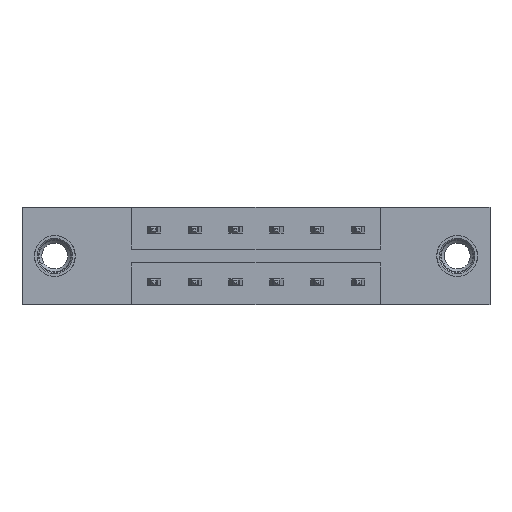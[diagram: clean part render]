
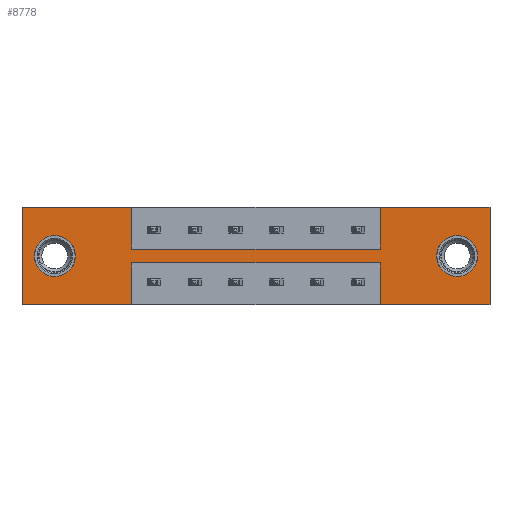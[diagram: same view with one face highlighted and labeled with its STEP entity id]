
A CAD part, front view. The second image highlights one B-rep face of the part: STEP entity #8778.
In plain terms, the highlighted planar face has unit normal (0, -1, 0).
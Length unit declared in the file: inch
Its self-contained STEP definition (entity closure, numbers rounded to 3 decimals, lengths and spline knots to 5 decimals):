
#43 = LINE ( 'NONE', #3060, #4409 ) ;
#208 = VECTOR ( 'NONE', #5693, 39.37008 ) ;
#381 = EDGE_CURVE ( 'NONE', #5767, #5441, #43, .T. ) ;
#435 = FACE_OUTER_BOUND ( 'NONE', #5698, .T. ) ;
#554 = LINE ( 'NONE', #6455, #8464 ) ;
#583 = AXIS2_PLACEMENT_3D ( 'NONE', #6669, #5352, #9686 ) ;
#607 = DIRECTION ( 'NONE',  ( 0., 1., 0. ) ) ;
#630 = CARTESIAN_POINT ( 'NONE',  ( 0., 0., 0. ) ) ;
#822 = ORIENTED_EDGE ( 'NONE', *, *, #4869, .T. ) ;
#967 = VECTOR ( 'NONE', #7931, 39.37008 ) ;
#1008 = AXIS2_PLACEMENT_3D ( 'NONE', #5091, #5903, #8939 ) ;
#1076 = CARTESIAN_POINT ( 'NONE',  ( 0., 0., -0.37 ) ) ;
#1120 = ORIENTED_EDGE ( 'NONE', *, *, #381, .F. ) ;
#1141 = DIRECTION ( 'NONE',  ( 1., 0., 0. ) ) ;
#1148 = LINE ( 'NONE', #6303, #4455 ) ;
#1151 = CARTESIAN_POINT ( 'NONE',  ( 1.3665, 0., -0.1585 ) ) ;
#1163 = CARTESIAN_POINT ( 'NONE',  ( 0.4175, 0., -0.1585 ) ) ;
#1263 = LINE ( 'NONE', #1163, #8132 ) ;
#1305 = VECTOR ( 'NONE', #8753, 39.37008 ) ;
#1425 = LINE ( 'NONE', #3141, #7980 ) ;
#1603 = VECTOR ( 'NONE', #7417, 39.37008 ) ;
#1613 = VERTEX_POINT ( 'NONE', #2608 ) ;
#1787 = VERTEX_POINT ( 'NONE', #630 ) ;
#1839 = CARTESIAN_POINT ( 'NONE',  ( 1.784, 0., -0.37 ) ) ;
#1968 = PLANE ( 'NONE',  #4619 ) ;
#2608 = CARTESIAN_POINT ( 'NONE',  ( 1.3665, 0., -0.1585 ) ) ;
#2634 = VECTOR ( 'NONE', #9454, 39.37008 ) ;
#2713 = CARTESIAN_POINT ( 'NONE',  ( 0., 0., -0.37 ) ) ;
#2823 = VERTEX_POINT ( 'NONE', #6062 ) ;
#2960 = EDGE_CURVE ( 'NONE', #6636, #5767, #1148, .T. ) ;
#3026 = CARTESIAN_POINT ( 'NONE',  ( 0.4175, 0., 0. ) ) ;
#3060 = CARTESIAN_POINT ( 'NONE',  ( 0.4175, 0., -0.2115 ) ) ;
#3124 = VERTEX_POINT ( 'NONE', #8231 ) ;
#3141 = CARTESIAN_POINT ( 'NONE',  ( 1.784, 0., 0. ) ) ;
#3235 = CARTESIAN_POINT ( 'NONE',  ( 0.4175, 0., -0.2115 ) ) ;
#3307 = DIRECTION ( 'NONE',  ( -1., 0., 0. ) ) ;
#3402 = CARTESIAN_POINT ( 'NONE',  ( 0., 0., 0. ) ) ;
#3451 = EDGE_LOOP ( 'NONE', ( #822, #3766 ) ) ;
#3481 = DIRECTION ( 'NONE',  ( 0., 0., 1. ) ) ;
#3496 = EDGE_CURVE ( 'NONE', #5668, #1787, #5848, .T. ) ;
#3550 = LINE ( 'NONE', #7162, #2634 ) ;
#3578 = DIRECTION ( 'NONE',  ( 0., 0., -1. ) ) ;
#3601 = ORIENTED_EDGE ( 'NONE', *, *, #7201, .F. ) ;
#3766 = ORIENTED_EDGE ( 'NONE', *, *, #4940, .T. ) ;
#3806 = EDGE_CURVE ( 'NONE', #1787, #6797, #4154, .T. ) ;
#3820 = CARTESIAN_POINT ( 'NONE',  ( 1.659, 0., -0.107 ) ) ;
#3928 = EDGE_CURVE ( 'NONE', #4126, #4663, #9031, .T. ) ;
#4056 = DIRECTION ( 'NONE',  ( 0., 0., -1. ) ) ;
#4126 = VERTEX_POINT ( 'NONE', #7000 ) ;
#4154 = LINE ( 'NONE', #3402, #1305 ) ;
#4203 = ORIENTED_EDGE ( 'NONE', *, *, #7881, .F. ) ;
#4241 = ORIENTED_EDGE ( 'NONE', *, *, #3806, .F. ) ;
#4319 = VERTEX_POINT ( 'NONE', #1839 ) ;
#4409 = VECTOR ( 'NONE', #3307, 39.37008 ) ;
#4455 = VECTOR ( 'NONE', #3481, 39.37008 ) ;
#4562 = ORIENTED_EDGE ( 'NONE', *, *, #3496, .F. ) ;
#4619 = AXIS2_PLACEMENT_3D ( 'NONE', #2713, #9515, #7173 ) ;
#4663 = VERTEX_POINT ( 'NONE', #3820 ) ;
#4869 = EDGE_CURVE ( 'NONE', #3124, #9203, #6033, .T. ) ;
#4935 = CARTESIAN_POINT ( 'NONE',  ( 0., 0., -0.37 ) ) ;
#4940 = EDGE_CURVE ( 'NONE', #9203, #3124, #6974, .T. ) ;
#4962 = CARTESIAN_POINT ( 'NONE',  ( 1.3665, 0., -0.37 ) ) ;
#4986 = ORIENTED_EDGE ( 'NONE', *, *, #8275, .F. ) ;
#5003 = CIRCLE ( 'NONE', #583, 0.078 ) ;
#5006 = VERTEX_POINT ( 'NONE', #6187 ) ;
#5091 = CARTESIAN_POINT ( 'NONE',  ( 0.125, 0., -0.185 ) ) ;
#5157 = ORIENTED_EDGE ( 'NONE', *, *, #7501, .T. ) ;
#5194 = EDGE_CURVE ( 'NONE', #6797, #2823, #6465, .T. ) ;
#5225 = ORIENTED_EDGE ( 'NONE', *, *, #8699, .F. ) ;
#5267 = CARTESIAN_POINT ( 'NONE',  ( 0., 0., 0. ) ) ;
#5352 = DIRECTION ( 'NONE',  ( 0., 1., 0. ) ) ;
#5441 = VERTEX_POINT ( 'NONE', #3235 ) ;
#5470 = CARTESIAN_POINT ( 'NONE',  ( 0.4175, 0., -0.1585 ) ) ;
#5647 = DIRECTION ( 'NONE',  ( 1., 0., 0. ) ) ;
#5668 = VERTEX_POINT ( 'NONE', #4935 ) ;
#5680 = CARTESIAN_POINT ( 'NONE',  ( 0.4175, 0., -0.37 ) ) ;
#5693 = DIRECTION ( 'NONE',  ( 0., 0., -1. ) ) ;
#5698 = EDGE_LOOP ( 'NONE', ( #6883, #6481, #3601, #4986, #7463, #6211, #7692, #4241, #4562, #5225, #4203, #1120 ) ) ;
#5767 = VERTEX_POINT ( 'NONE', #9511 ) ;
#5848 = LINE ( 'NONE', #5267, #1603 ) ;
#5858 = DIRECTION ( 'NONE',  ( 0., 0., 1. ) ) ;
#5903 = DIRECTION ( 'NONE',  ( 0., 1., 0. ) ) ;
#5970 = DIRECTION ( 'NONE',  ( 0., 0., -1. ) ) ;
#6025 = CARTESIAN_POINT ( 'NONE',  ( 1.659, 0., -0.185 ) ) ;
#6033 = CIRCLE ( 'NONE', #9514, 0.078 ) ;
#6062 = CARTESIAN_POINT ( 'NONE',  ( 0.4175, 0., -0.1585 ) ) ;
#6187 = CARTESIAN_POINT ( 'NONE',  ( 1.3665, 0., 0. ) ) ;
#6211 = ORIENTED_EDGE ( 'NONE', *, *, #7389, .F. ) ;
#6303 = CARTESIAN_POINT ( 'NONE',  ( 1.3665, 0., -0.2115 ) ) ;
#6318 = AXIS2_PLACEMENT_3D ( 'NONE', #6025, #607, #5970 ) ;
#6433 = LINE ( 'NONE', #1076, #967 ) ;
#6455 = CARTESIAN_POINT ( 'NONE',  ( 0.4175, 0., -0.2115 ) ) ;
#6465 = LINE ( 'NONE', #5470, #208 ) ;
#6481 = ORIENTED_EDGE ( 'NONE', *, *, #7337, .F. ) ;
#6536 = CARTESIAN_POINT ( 'NONE',  ( 0.125, 0., -0.185 ) ) ;
#6601 = EDGE_CURVE ( 'NONE', #1613, #5006, #7903, .T. ) ;
#6636 = VERTEX_POINT ( 'NONE', #4962 ) ;
#6669 = CARTESIAN_POINT ( 'NONE',  ( 1.659, 0., -0.185 ) ) ;
#6691 = DIRECTION ( 'NONE',  ( 0., 1., 0. ) ) ;
#6797 = VERTEX_POINT ( 'NONE', #3026 ) ;
#6883 = ORIENTED_EDGE ( 'NONE', *, *, #2960, .F. ) ;
#6974 = CIRCLE ( 'NONE', #1008, 0.078 ) ;
#7000 = CARTESIAN_POINT ( 'NONE',  ( 1.659, 0., -0.263 ) ) ;
#7070 = FACE_BOUND ( 'NONE', #3451, .T. ) ;
#7083 = LINE ( 'NONE', #8783, #9254 ) ;
#7162 = CARTESIAN_POINT ( 'NONE',  ( 0., 0., -0.37 ) ) ;
#7173 = DIRECTION ( 'NONE',  ( 0., 0., -1. ) ) ;
#7174 = EDGE_LOOP ( 'NONE', ( #5157, #7415 ) ) ;
#7201 = EDGE_CURVE ( 'NONE', #8276, #4319, #1425, .T. ) ;
#7337 = EDGE_CURVE ( 'NONE', #4319, #6636, #3550, .T. ) ;
#7389 = EDGE_CURVE ( 'NONE', #2823, #1613, #1263, .T. ) ;
#7415 = ORIENTED_EDGE ( 'NONE', *, *, #3928, .T. ) ;
#7417 = DIRECTION ( 'NONE',  ( 0., 0., 1. ) ) ;
#7463 = ORIENTED_EDGE ( 'NONE', *, *, #6601, .F. ) ;
#7501 = EDGE_CURVE ( 'NONE', #4663, #4126, #5003, .T. ) ;
#7692 = ORIENTED_EDGE ( 'NONE', *, *, #5194, .F. ) ;
#7817 = VERTEX_POINT ( 'NONE', #5680 ) ;
#7881 = EDGE_CURVE ( 'NONE', #5441, #7817, #554, .T. ) ;
#7903 = LINE ( 'NONE', #1151, #8437 ) ;
#7931 = DIRECTION ( 'NONE',  ( -1., 0., 0. ) ) ;
#7980 = VECTOR ( 'NONE', #4056, 39.37008 ) ;
#8132 = VECTOR ( 'NONE', #5647, 39.37008 ) ;
#8231 = CARTESIAN_POINT ( 'NONE',  ( 0.125, 0., -0.107 ) ) ;
#8275 = EDGE_CURVE ( 'NONE', #5006, #8276, #7083, .T. ) ;
#8276 = VERTEX_POINT ( 'NONE', #9476 ) ;
#8437 = VECTOR ( 'NONE', #8748, 39.37008 ) ;
#8464 = VECTOR ( 'NONE', #3578, 39.37008 ) ;
#8699 = EDGE_CURVE ( 'NONE', #7817, #5668, #6433, .T. ) ;
#8748 = DIRECTION ( 'NONE',  ( 0., 0., 1. ) ) ;
#8753 = DIRECTION ( 'NONE',  ( 1., 0., 0. ) ) ;
#8778 = ADVANCED_FACE ( 'NONE', ( #9328, #7070, #435 ), #1968, .T. ) ;
#8783 = CARTESIAN_POINT ( 'NONE',  ( 0., 0., 0. ) ) ;
#8939 = DIRECTION ( 'NONE',  ( 0., 0., 1. ) ) ;
#9031 = CIRCLE ( 'NONE', #6318, 0.078 ) ;
#9203 = VERTEX_POINT ( 'NONE', #9395 ) ;
#9254 = VECTOR ( 'NONE', #1141, 39.37008 ) ;
#9328 = FACE_BOUND ( 'NONE', #7174, .T. ) ;
#9395 = CARTESIAN_POINT ( 'NONE',  ( 0.125, 0., -0.263 ) ) ;
#9454 = DIRECTION ( 'NONE',  ( -1., 0., 0. ) ) ;
#9476 = CARTESIAN_POINT ( 'NONE',  ( 1.784, 0., 0. ) ) ;
#9511 = CARTESIAN_POINT ( 'NONE',  ( 1.3665, 0., -0.2115 ) ) ;
#9514 = AXIS2_PLACEMENT_3D ( 'NONE', #6536, #6691, #5858 ) ;
#9515 = DIRECTION ( 'NONE',  ( 0., -1., 0. ) ) ;
#9686 = DIRECTION ( 'NONE',  ( 0., 0., -1. ) ) ;
